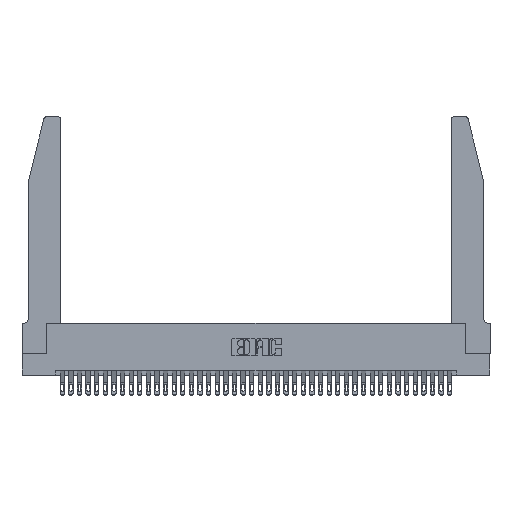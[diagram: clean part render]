
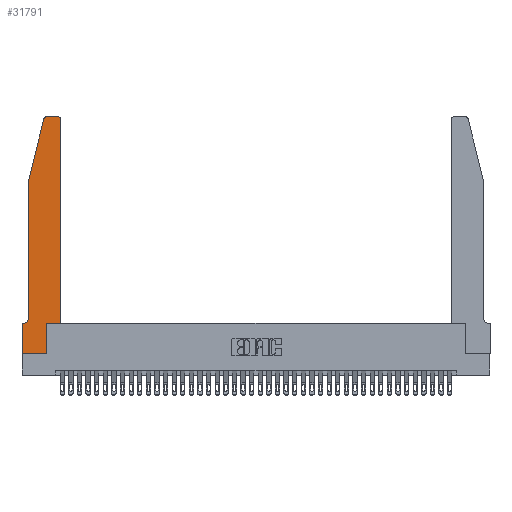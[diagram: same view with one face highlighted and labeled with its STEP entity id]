
A CAD part, top view. The second image highlights one B-rep face of the part: STEP entity #31791.
In plain terms, the highlighted planar face has unit normal (0, 0, 1).
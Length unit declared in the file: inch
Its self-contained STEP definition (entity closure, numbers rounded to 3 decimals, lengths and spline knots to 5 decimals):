
#534 = VERTEX_POINT ( 'NONE', #20796 ) ;
#1130 = CARTESIAN_POINT ( 'NONE',  ( 0.2865, 0.35, 0.37 ) ) ;
#1256 = EDGE_CURVE ( 'NONE', #23625, #14892, #23254, .T. ) ;
#1285 = ORIENTED_EDGE ( 'NONE', *, *, #32336, .T. ) ;
#1450 = EDGE_CURVE ( 'NONE', #8817, #35978, #38386, .T. ) ;
#2059 = DIRECTION ( 'NONE',  ( 1., 0., 0. ) ) ;
#2678 = VERTEX_POINT ( 'NONE', #6579 ) ;
#2724 = CARTESIAN_POINT ( 'NONE',  ( 0.0755, 2., 0.37 ) ) ;
#2973 = CARTESIAN_POINT ( 'NONE',  ( 0.4505, 2.72, 0.37 ) ) ;
#3060 = EDGE_CURVE ( 'NONE', #2678, #9015, #10818, .T. ) ;
#3571 = VECTOR ( 'NONE', #17322, 39.37008 ) ;
#3583 = EDGE_CURVE ( 'NONE', #9015, #12868, #4408, .T. ) ;
#3865 = VECTOR ( 'NONE', #38935, 39.37008 ) ;
#4408 = LINE ( 'NONE', #28545, #40294 ) ;
#4413 = DIRECTION ( 'NONE',  ( -1., 0., 0. ) ) ;
#4967 = DIRECTION ( 'NONE',  ( 0., 0., 1. ) ) ;
#5247 = ORIENTED_EDGE ( 'NONE', *, *, #40081, .T. ) ;
#6566 = DIRECTION ( 'NONE',  ( -1., 0., 0. ) ) ;
#6579 = CARTESIAN_POINT ( 'NONE',  ( 0.0055, 0.35, 0.37 ) ) ;
#7149 = LINE ( 'NONE', #1130, #30229 ) ;
#7544 = ORIENTED_EDGE ( 'NONE', *, *, #1256, .T. ) ;
#8251 = PLANE ( 'NONE',  #28494 ) ;
#8678 = ORIENTED_EDGE ( 'NONE', *, *, #11733, .T. ) ;
#8817 = VERTEX_POINT ( 'NONE', #2973 ) ;
#8946 = EDGE_CURVE ( 'NONE', #35978, #12444, #24372, .T. ) ;
#9015 = VERTEX_POINT ( 'NONE', #36051 ) ;
#9173 = DIRECTION ( 'NONE',  ( 1., 0., 0. ) ) ;
#9687 = EDGE_CURVE ( 'NONE', #12868, #15636, #31360, .T. ) ;
#10562 = CARTESIAN_POINT ( 'NONE',  ( 0.0055, 0.42, 0.37 ) ) ;
#10818 = LINE ( 'NONE', #31741, #34917 ) ;
#11091 = ORIENTED_EDGE ( 'NONE', *, *, #23670, .T. ) ;
#11209 = LINE ( 'NONE', #14406, #13186 ) ;
#11658 = VECTOR ( 'NONE', #27532, 39.37008 ) ;
#11733 = EDGE_CURVE ( 'NONE', #15636, #534, #7149, .T. ) ;
#12444 = VERTEX_POINT ( 'NONE', #21017 ) ;
#12499 = CARTESIAN_POINT ( 'NONE',  ( 0., 0., 0.37 ) ) ;
#12868 = VERTEX_POINT ( 'NONE', #13227 ) ;
#13186 = VECTOR ( 'NONE', #36370, 39.37008 ) ;
#13227 = CARTESIAN_POINT ( 'NONE',  ( 0., 0., 0.37 ) ) ;
#13435 = DIRECTION ( 'NONE',  ( 0., 0., -1. ) ) ;
#14406 = CARTESIAN_POINT ( 'NONE',  ( 0.4505, 0.35, 0.37 ) ) ;
#14558 = DIRECTION ( 'NONE',  ( 0., 0., 1. ) ) ;
#14892 = VERTEX_POINT ( 'NONE', #2724 ) ;
#15636 = VERTEX_POINT ( 'NONE', #17314 ) ;
#15826 = CARTESIAN_POINT ( 'NONE',  ( 0.4505, 0.35, 0.37 ) ) ;
#15973 = CIRCLE ( 'NONE', #21414, 0.07 ) ;
#15981 = EDGE_LOOP ( 'NONE', ( #35800, #11091, #7544, #27995, #1285, #17207, #34993, #38923, #8678, #5247, #37254, #29818 ) ) ;
#16001 = VECTOR ( 'NONE', #6566, 39.37008 ) ;
#16009 = FACE_OUTER_BOUND ( 'NONE', #15981, .T. ) ;
#17182 = CARTESIAN_POINT ( 'NONE',  ( 0.4205, 2.72, 0.37 ) ) ;
#17207 = ORIENTED_EDGE ( 'NONE', *, *, #3060, .T. ) ;
#17299 = CIRCLE ( 'NONE', #26932, 0.03 ) ;
#17314 = CARTESIAN_POINT ( 'NONE',  ( 0.2865, 0., 0.37 ) ) ;
#17322 = DIRECTION ( 'NONE',  ( -0.239, -0.971, 0. ) ) ;
#17344 = DIRECTION ( 'NONE',  ( 0., 0., 1. ) ) ;
#18266 = CARTESIAN_POINT ( 'NONE',  ( 0.284, 2.72, 0.37 ) ) ;
#20404 = VERTEX_POINT ( 'NONE', #32551 ) ;
#20796 = CARTESIAN_POINT ( 'NONE',  ( 0.2865, 0.35, 0.37 ) ) ;
#20990 = VECTOR ( 'NONE', #38155, 39.37008 ) ;
#21017 = CARTESIAN_POINT ( 'NONE',  ( 0.284, 2.75, 0.37 ) ) ;
#21414 = AXIS2_PLACEMENT_3D ( 'NONE', #10562, #13435, #4413 ) ;
#21998 = LINE ( 'NONE', #15826, #20990 ) ;
#23020 = LINE ( 'NONE', #33716, #11658 ) ;
#23254 = LINE ( 'NONE', #33520, #3571 ) ;
#23625 = VERTEX_POINT ( 'NONE', #24133 ) ;
#23670 = EDGE_CURVE ( 'NONE', #12444, #23625, #17299, .T. ) ;
#24133 = CARTESIAN_POINT ( 'NONE',  ( 0.25487, 2.72718, 0.37 ) ) ;
#24372 = LINE ( 'NONE', #34712, #16001 ) ;
#24724 = CARTESIAN_POINT ( 'NONE',  ( 0.0755, 0.42, 0.37 ) ) ;
#26932 = AXIS2_PLACEMENT_3D ( 'NONE', #18266, #14558, #9173 ) ;
#27532 = DIRECTION ( 'NONE',  ( 0., -1., 0. ) ) ;
#27995 = ORIENTED_EDGE ( 'NONE', *, *, #30120, .T. ) ;
#28494 = AXIS2_PLACEMENT_3D ( 'NONE', #39433, #17344, #36431 ) ;
#28545 = CARTESIAN_POINT ( 'NONE',  ( 0., 0., 0.37 ) ) ;
#29068 = DIRECTION ( 'NONE',  ( 0., -1., 0. ) ) ;
#29499 = EDGE_CURVE ( 'NONE', #20404, #8817, #11209, .T. ) ;
#29818 = ORIENTED_EDGE ( 'NONE', *, *, #1450, .T. ) ;
#30120 = EDGE_CURVE ( 'NONE', #14892, #37285, #23020, .T. ) ;
#30229 = VECTOR ( 'NONE', #32890, 39.37008 ) ;
#30612 = DIRECTION ( 'NONE',  ( -1., 0., 0. ) ) ;
#31360 = LINE ( 'NONE', #12499, #3865 ) ;
#31720 = CARTESIAN_POINT ( 'NONE',  ( 0.4205, 2.75, 0.37 ) ) ;
#31741 = CARTESIAN_POINT ( 'NONE',  ( 0.0755, 0.35, 0.37 ) ) ;
#31791 = ADVANCED_FACE ( 'NONE', ( #16009 ), #8251, .T. ) ;
#32137 = AXIS2_PLACEMENT_3D ( 'NONE', #17182, #4967, #2059 ) ;
#32336 = EDGE_CURVE ( 'NONE', #37285, #2678, #15973, .T. ) ;
#32551 = CARTESIAN_POINT ( 'NONE',  ( 0.4505, 0.35, 0.37 ) ) ;
#32890 = DIRECTION ( 'NONE',  ( 0., 1., 0. ) ) ;
#33520 = CARTESIAN_POINT ( 'NONE',  ( 0.0755, 2., 0.37 ) ) ;
#33716 = CARTESIAN_POINT ( 'NONE',  ( 0.0755, 2., 0.37 ) ) ;
#34712 = CARTESIAN_POINT ( 'NONE',  ( 0.2605, 2.75, 0.37 ) ) ;
#34917 = VECTOR ( 'NONE', #30612, 39.37008 ) ;
#34993 = ORIENTED_EDGE ( 'NONE', *, *, #3583, .T. ) ;
#35800 = ORIENTED_EDGE ( 'NONE', *, *, #8946, .T. ) ;
#35978 = VERTEX_POINT ( 'NONE', #31720 ) ;
#36051 = CARTESIAN_POINT ( 'NONE',  ( 0., 0.35, 0.37 ) ) ;
#36370 = DIRECTION ( 'NONE',  ( 0., 1., 0. ) ) ;
#36431 = DIRECTION ( 'NONE',  ( 1., 0., 0. ) ) ;
#37254 = ORIENTED_EDGE ( 'NONE', *, *, #29499, .T. ) ;
#37285 = VERTEX_POINT ( 'NONE', #24724 ) ;
#38155 = DIRECTION ( 'NONE',  ( 1., 0., 0. ) ) ;
#38386 = CIRCLE ( 'NONE', #32137, 0.03 ) ;
#38923 = ORIENTED_EDGE ( 'NONE', *, *, #9687, .T. ) ;
#38935 = DIRECTION ( 'NONE',  ( 1., 0., 0. ) ) ;
#39433 = CARTESIAN_POINT ( 'NONE',  ( 0., 0.35, 0.37 ) ) ;
#40081 = EDGE_CURVE ( 'NONE', #534, #20404, #21998, .T. ) ;
#40294 = VECTOR ( 'NONE', #29068, 39.37008 ) ;
